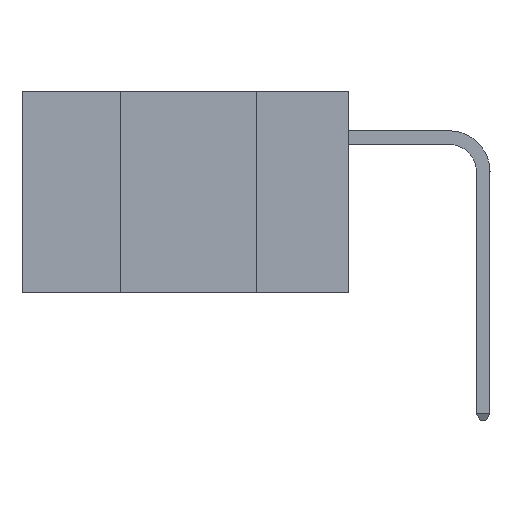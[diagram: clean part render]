
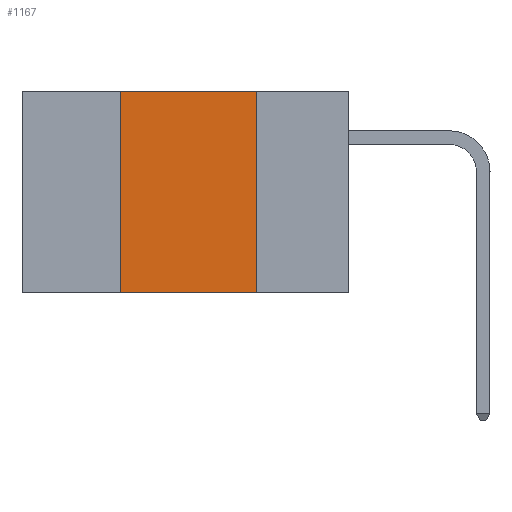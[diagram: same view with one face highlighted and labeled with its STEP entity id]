
A CAD part, left-side view. The second image highlights one B-rep face of the part: STEP entity #1167.
In plain terms, the highlighted planar face has unit normal (-1, 0, 0).
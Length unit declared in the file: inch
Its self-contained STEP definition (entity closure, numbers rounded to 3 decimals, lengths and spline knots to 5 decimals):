
#98 = FACE_OUTER_BOUND ( 'NONE', #7668, .T. ) ;
#103 = ORIENTED_EDGE ( 'NONE', *, *, #6763, .F. ) ;
#268 = ORIENTED_EDGE ( 'NONE', *, *, #5740, .F. ) ;
#328 = ORIENTED_EDGE ( 'NONE', *, *, #10822, .F. ) ;
#371 = ORIENTED_EDGE ( 'NONE', *, *, #9129, .T. ) ;
#382 = LINE ( 'NONE', #3791, #10432 ) ;
#931 = CARTESIAN_POINT ( 'NONE',  ( 0., 0.6, -0.37 ) ) ;
#1137 = CARTESIAN_POINT ( 'NONE',  ( 0., 0.6, 0. ) ) ;
#1167 = ADVANCED_FACE ( 'NONE', ( #98 ), #1950, .F. ) ;
#1780 = VERTEX_POINT ( 'NONE', #3698 ) ;
#1894 = DIRECTION ( 'NONE',  ( 0., -1., 0. ) ) ;
#1950 = PLANE ( 'NONE',  #6550 ) ;
#1959 = DIRECTION ( 'NONE',  ( 0., 0., -1. ) ) ;
#2736 = LINE ( 'NONE', #9458, #7235 ) ;
#3698 = CARTESIAN_POINT ( 'NONE',  ( 0., 0.42, -0.37 ) ) ;
#3791 = CARTESIAN_POINT ( 'NONE',  ( 0., 0.42, 0. ) ) ;
#4200 = VERTEX_POINT ( 'NONE', #12160 ) ;
#4753 = DIRECTION ( 'NONE',  ( 0., 0., -1. ) ) ;
#4965 = VECTOR ( 'NONE', #12517, 39.37008 ) ;
#5740 = EDGE_CURVE ( 'NONE', #4200, #8989, #7414, .T. ) ;
#6259 = VERTEX_POINT ( 'NONE', #10403 ) ;
#6550 = AXIS2_PLACEMENT_3D ( 'NONE', #1137, #7412, #1959 ) ;
#6704 = CARTESIAN_POINT ( 'NONE',  ( 0., 0.6, 0. ) ) ;
#6763 = EDGE_CURVE ( 'NONE', #8989, #6259, #2736, .T. ) ;
#7235 = VECTOR ( 'NONE', #4753, 39.37008 ) ;
#7412 = DIRECTION ( 'NONE',  ( 1., 0., 0. ) ) ;
#7414 = LINE ( 'NONE', #6704, #11597 ) ;
#7668 = EDGE_LOOP ( 'NONE', ( #103, #268, #328, #371 ) ) ;
#8989 = VERTEX_POINT ( 'NONE', #11366 ) ;
#9129 = EDGE_CURVE ( 'NONE', #1780, #6259, #10013, .T. ) ;
#9453 = DIRECTION ( 'NONE',  ( 0., 0., 1. ) ) ;
#9458 = CARTESIAN_POINT ( 'NONE',  ( 0., 0.17, 0. ) ) ;
#10013 = LINE ( 'NONE', #931, #4965 ) ;
#10403 = CARTESIAN_POINT ( 'NONE',  ( 0., 0.17, -0.37 ) ) ;
#10432 = VECTOR ( 'NONE', #9453, 39.37008 ) ;
#10822 = EDGE_CURVE ( 'NONE', #1780, #4200, #382, .T. ) ;
#11366 = CARTESIAN_POINT ( 'NONE',  ( 0., 0.17, 0. ) ) ;
#11597 = VECTOR ( 'NONE', #1894, 39.37008 ) ;
#12160 = CARTESIAN_POINT ( 'NONE',  ( 0., 0.42, 0. ) ) ;
#12517 = DIRECTION ( 'NONE',  ( 0., -1., 0. ) ) ;
